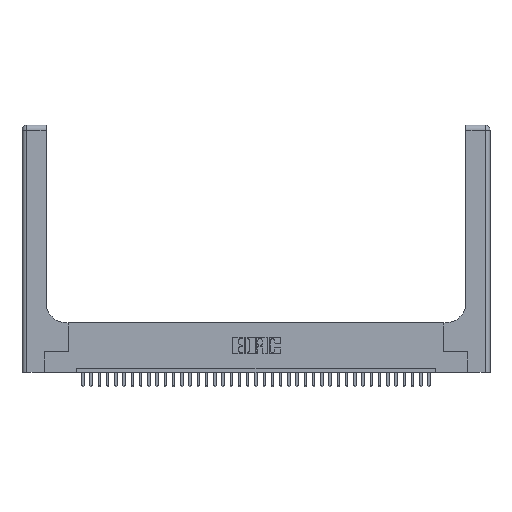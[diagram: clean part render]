
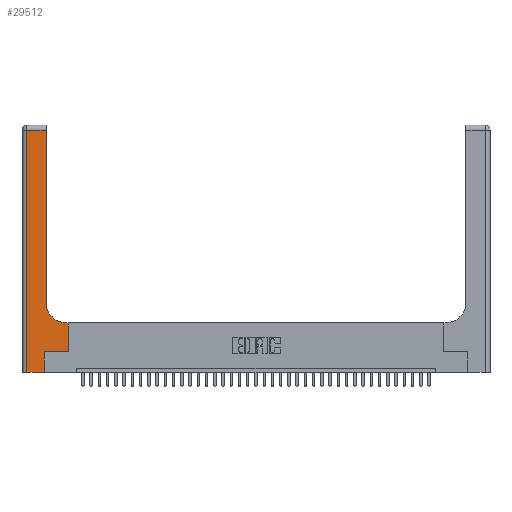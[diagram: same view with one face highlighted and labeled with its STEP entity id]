
A CAD part, top view. The second image highlights one B-rep face of the part: STEP entity #29512.
In plain terms, the highlighted planar face has unit normal (0, 0, 1).
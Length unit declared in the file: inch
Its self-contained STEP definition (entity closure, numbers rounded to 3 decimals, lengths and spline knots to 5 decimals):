
#311 = AXIS2_PLACEMENT_3D ( 'NONE', #30061, #4509, #35940 ) ;
#563 = CARTESIAN_POINT ( 'NONE',  ( 0.269, 0., 0.37 ) ) ;
#928 = LINE ( 'NONE', #29213, #34019 ) ;
#1978 = DIRECTION ( 'NONE',  ( 0., 1., 0. ) ) ;
#2149 = VECTOR ( 'NONE', #18735, 39.37008 ) ;
#2252 = EDGE_CURVE ( 'NONE', #26617, #22393, #928, .T. ) ;
#2608 = LINE ( 'NONE', #7659, #32429 ) ;
#3058 = CARTESIAN_POINT ( 'NONE',  ( 0.269, 0.25, 0.37 ) ) ;
#3091 = ORIENTED_EDGE ( 'NONE', *, *, #20056, .T. ) ;
#4245 = DIRECTION ( 'NONE',  ( 0., -1., 0. ) ) ;
#4509 = DIRECTION ( 'NONE',  ( 0., 0., -1. ) ) ;
#4688 = CARTESIAN_POINT ( 'NONE',  ( 0.5585, 0.25, 0.37 ) ) ;
#5053 = CARTESIAN_POINT ( 'NONE',  ( 0.2915, 2.94, 0.37 ) ) ;
#5726 = VERTEX_POINT ( 'NONE', #17512 ) ;
#5778 = CARTESIAN_POINT ( 'NONE',  ( 0., 2.94, 0.37 ) ) ;
#7209 = EDGE_CURVE ( 'NONE', #5726, #19532, #10686, .T. ) ;
#7659 = CARTESIAN_POINT ( 'NONE',  ( 0.2915, 0.6, 0.37 ) ) ;
#7999 = CARTESIAN_POINT ( 'NONE',  ( 0.269, 0.25, 0.37 ) ) ;
#8275 = DIRECTION ( 'NONE',  ( 1., 0., 0. ) ) ;
#8620 = DIRECTION ( 'NONE',  ( 0., 1., 0. ) ) ;
#8918 = DIRECTION ( 'NONE',  ( 0., 1., 0. ) ) ;
#9303 = LINE ( 'NONE', #7999, #24696 ) ;
#10062 = CARTESIAN_POINT ( 'NONE',  ( 0.06, 3., 0.37 ) ) ;
#10582 = FACE_OUTER_BOUND ( 'NONE', #30502, .T. ) ;
#10614 = LINE ( 'NONE', #5778, #24149 ) ;
#10686 = LINE ( 'NONE', #30020, #2149 ) ;
#10735 = ORIENTED_EDGE ( 'NONE', *, *, #2252, .T. ) ;
#11981 = VERTEX_POINT ( 'NONE', #3058 ) ;
#12053 = LINE ( 'NONE', #28952, #30712 ) ;
#13304 = ORIENTED_EDGE ( 'NONE', *, *, #29292, .T. ) ;
#13439 = ORIENTED_EDGE ( 'NONE', *, *, #7209, .T. ) ;
#16800 = DIRECTION ( 'NONE',  ( 1., 0., 0. ) ) ;
#17512 = CARTESIAN_POINT ( 'NONE',  ( 0.06, 0., 0.37 ) ) ;
#18250 = CARTESIAN_POINT ( 'NONE',  ( 0.06, 2.94, 0.37 ) ) ;
#18329 = LINE ( 'NONE', #563, #31961 ) ;
#18735 = DIRECTION ( 'NONE',  ( 1., 0., 0. ) ) ;
#18998 = VERTEX_POINT ( 'NONE', #27758 ) ;
#19026 = PLANE ( 'NONE',  #311 ) ;
#19532 = VERTEX_POINT ( 'NONE', #22935 ) ;
#20056 = EDGE_CURVE ( 'NONE', #22393, #32985, #2608, .T. ) ;
#21356 = CARTESIAN_POINT ( 'NONE',  ( 0.5585, 0.6, 0.37 ) ) ;
#22393 = VERTEX_POINT ( 'NONE', #21356 ) ;
#22935 = CARTESIAN_POINT ( 'NONE',  ( 0.269, 0., 0.37 ) ) ;
#23097 = ORIENTED_EDGE ( 'NONE', *, *, #23105, .T. ) ;
#23105 = EDGE_CURVE ( 'NONE', #18998, #27037, #12053, .T. ) ;
#23164 = DIRECTION ( 'NONE',  ( -1., 0., 0. ) ) ;
#24114 = EDGE_CURVE ( 'NONE', #19532, #11981, #18329, .T. ) ;
#24149 = VECTOR ( 'NONE', #23164, 39.37008 ) ;
#24270 = VERTEX_POINT ( 'NONE', #18250 ) ;
#24538 = ORIENTED_EDGE ( 'NONE', *, *, #33739, .T. ) ;
#24613 = ORIENTED_EDGE ( 'NONE', *, *, #27584, .T. ) ;
#24696 = VECTOR ( 'NONE', #16800, 39.37008 ) ;
#25218 = DIRECTION ( 'NONE',  ( 0., 0., -1. ) ) ;
#26617 = VERTEX_POINT ( 'NONE', #4688 ) ;
#26690 = AXIS2_PLACEMENT_3D ( 'NONE', #28138, #25218, #8275 ) ;
#27037 = VERTEX_POINT ( 'NONE', #5053 ) ;
#27584 = EDGE_CURVE ( 'NONE', #32985, #18998, #30832, .T. ) ;
#27758 = CARTESIAN_POINT ( 'NONE',  ( 0.2915, 0.85, 0.37 ) ) ;
#28138 = CARTESIAN_POINT ( 'NONE',  ( 0.5415, 0.85, 0.37 ) ) ;
#28952 = CARTESIAN_POINT ( 'NONE',  ( 0.2915, 3., 0.37 ) ) ;
#29213 = CARTESIAN_POINT ( 'NONE',  ( 0.5585, 0.25, 0.37 ) ) ;
#29292 = EDGE_CURVE ( 'NONE', #27037, #24270, #10614, .T. ) ;
#29512 = ADVANCED_FACE ( 'NONE', ( #10582 ), #19026, .F. ) ;
#29514 = DIRECTION ( 'NONE',  ( -1., 0., 0. ) ) ;
#29773 = LINE ( 'NONE', #10062, #33453 ) ;
#30020 = CARTESIAN_POINT ( 'NONE',  ( 0., 0., 0.37 ) ) ;
#30061 = CARTESIAN_POINT ( 'NONE',  ( 0., 3., 0.37 ) ) ;
#30502 = EDGE_LOOP ( 'NONE', ( #23097, #13304, #37199, #13439, #36832, #24538, #10735, #3091, #24613 ) ) ;
#30712 = VECTOR ( 'NONE', #1978, 39.37008 ) ;
#30832 = CIRCLE ( 'NONE', #26690, 0.25 ) ;
#31961 = VECTOR ( 'NONE', #8918, 39.37008 ) ;
#32429 = VECTOR ( 'NONE', #29514, 39.37008 ) ;
#32985 = VERTEX_POINT ( 'NONE', #33226 ) ;
#33226 = CARTESIAN_POINT ( 'NONE',  ( 0.5415, 0.6, 0.37 ) ) ;
#33453 = VECTOR ( 'NONE', #4245, 39.37008 ) ;
#33739 = EDGE_CURVE ( 'NONE', #11981, #26617, #9303, .T. ) ;
#34019 = VECTOR ( 'NONE', #8620, 39.37008 ) ;
#35940 = DIRECTION ( 'NONE',  ( -1., 0., 0. ) ) ;
#36552 = EDGE_CURVE ( 'NONE', #24270, #5726, #29773, .T. ) ;
#36832 = ORIENTED_EDGE ( 'NONE', *, *, #24114, .T. ) ;
#37199 = ORIENTED_EDGE ( 'NONE', *, *, #36552, .T. ) ;
